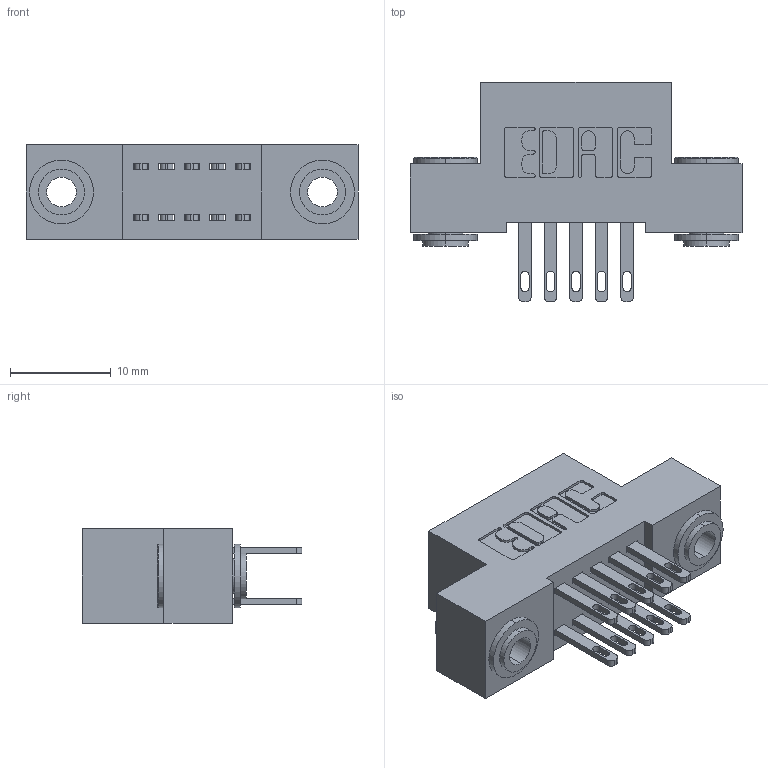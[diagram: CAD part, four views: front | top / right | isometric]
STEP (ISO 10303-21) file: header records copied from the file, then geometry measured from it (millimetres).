
FILE_DESCRIPTION (( 'STEP AP203' ), '1' );
FILE_NAME ('892-010-500-203.STEP', '2020-09-21T12:50:33', ( '' ), ( '' ), 'SwSTEP 2.0', 'SolidWorks 2020', '' );
FILE_SCHEMA (( 'CONFIG_CONTROL_DESIGN' ));
Length unit declared in the file: inch
Products named in the file (4): 892-010-500-203; 345-292-001_345-293-100; 842 Part_.156 TH; 342-250-002_345-250-002-102
Assembly tree (13 placements, depth 2):
  892-010-500-203
    842 Part_.156 TH
    345-292-001_345-293-100  x10
    342-250-002_345-250-002-102  x2
Bounding box: 33.02 x 21.85 x 9.4 mm (x, y, z)
Volume: 2845.1 mm3; surface area: 4029.2 mm2
Topology: 13 solids, 13 shells, 628 faces, 1845 edges, 1226 vertices
Faces by surface type: plane 376, cylinder 244, cone 8
Entity records: 8450 total; most frequent: CARTESIAN_POINT 1417, ORIENTED_EDGE 1346, DIRECTION 1311, EDGE_CURVE 673, LINE 517, VECTOR 517, VERTEX_POINT 446, AXIS2_PLACEMENT_3D 397
